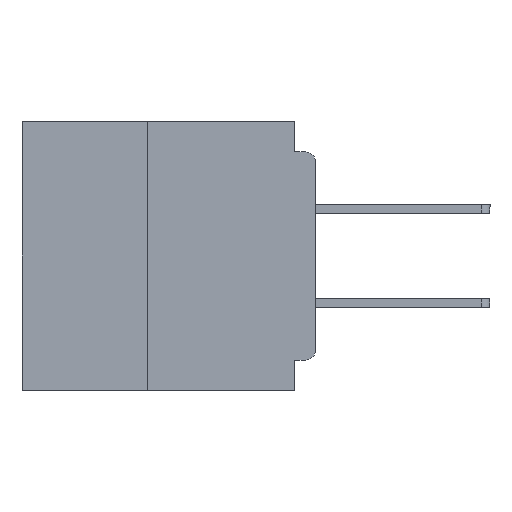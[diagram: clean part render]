
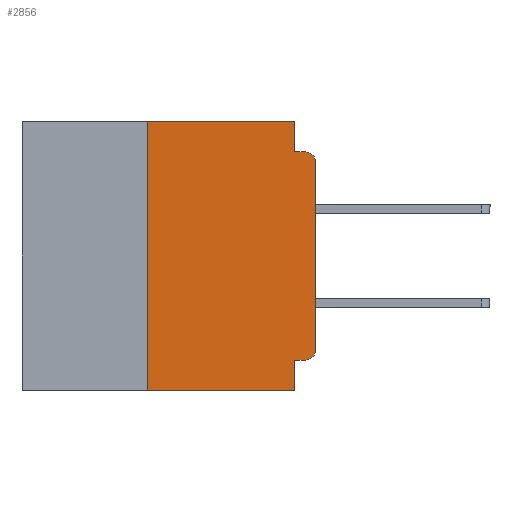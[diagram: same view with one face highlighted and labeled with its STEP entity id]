
A CAD part, left-side view. The second image highlights one B-rep face of the part: STEP entity #2856.
In plain terms, the highlighted planar face has unit normal (-1, 0, 0).
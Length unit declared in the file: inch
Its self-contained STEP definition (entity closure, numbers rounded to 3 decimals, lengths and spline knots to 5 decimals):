
#114 = CARTESIAN_POINT ( 'NONE',  ( 0., 0., 0. ) ) ;
#405 = EDGE_CURVE ( 'NONE', #44280, #7574, #28032, .T. ) ;
#1463 = EDGE_CURVE ( 'NONE', #37430, #23000, #16809, .T. ) ;
#2171 = DIRECTION ( 'NONE',  ( 0., 0., -1. ) ) ;
#2645 = CARTESIAN_POINT ( 'NONE',  ( 0., 0., -0.045 ) ) ;
#2856 = ADVANCED_FACE ( 'NONE', ( #10744 ), #32608, .F. ) ;
#2938 = EDGE_CURVE ( 'NONE', #18710, #21961, #27287, .T. ) ;
#4623 = CIRCLE ( 'NONE', #25023, 0.015 ) ;
#4988 = CARTESIAN_POINT ( 'NONE',  ( 0., 0.437, 0. ) ) ;
#5082 = CARTESIAN_POINT ( 'NONE',  ( 0., 0.015, -0.355 ) ) ;
#5826 = LINE ( 'NONE', #114, #45745 ) ;
#6076 = ORIENTED_EDGE ( 'NONE', *, *, #46661, .T. ) ;
#6151 = LINE ( 'NONE', #39834, #42581 ) ;
#6494 = CARTESIAN_POINT ( 'NONE',  ( 0., 0., -0.355 ) ) ;
#6638 = ORIENTED_EDGE ( 'NONE', *, *, #2938, .F. ) ;
#7228 = VECTOR ( 'NONE', #45148, 39.37008 ) ;
#7574 = VERTEX_POINT ( 'NONE', #24843 ) ;
#7964 = VERTEX_POINT ( 'NONE', #11908 ) ;
#7988 = VECTOR ( 'NONE', #12850, 39.37008 ) ;
#8769 = DIRECTION ( 'NONE',  ( 0., -1., 0. ) ) ;
#10744 = FACE_OUTER_BOUND ( 'NONE', #28054, .T. ) ;
#10746 = ORIENTED_EDGE ( 'NONE', *, *, #1463, .F. ) ;
#10766 = CARTESIAN_POINT ( 'NONE',  ( 0., 0.015, -0.06 ) ) ;
#10974 = LINE ( 'NONE', #35877, #28697 ) ;
#11908 = CARTESIAN_POINT ( 'NONE',  ( 0., 0., -0.34 ) ) ;
#11977 = VERTEX_POINT ( 'NONE', #30404 ) ;
#12850 = DIRECTION ( 'NONE',  ( 0., 0., 1. ) ) ;
#12955 = CARTESIAN_POINT ( 'NONE',  ( 0., 0.031, -0.355 ) ) ;
#13280 = DIRECTION ( 'NONE',  ( 0., -1., 0. ) ) ;
#13637 = ORIENTED_EDGE ( 'NONE', *, *, #16583, .F. ) ;
#13921 = VECTOR ( 'NONE', #36580, 39.37008 ) ;
#14238 = CARTESIAN_POINT ( 'NONE',  ( 0., 0.031, 0. ) ) ;
#14565 = DIRECTION ( 'NONE',  ( 0., 0., -1. ) ) ;
#16583 = EDGE_CURVE ( 'NONE', #21961, #11977, #24001, .T. ) ;
#16809 = LINE ( 'NONE', #6494, #35683 ) ;
#18105 = LINE ( 'NONE', #4988, #46826 ) ;
#18710 = VERTEX_POINT ( 'NONE', #14238 ) ;
#19226 = VERTEX_POINT ( 'NONE', #39712 ) ;
#21714 = DIRECTION ( 'NONE',  ( -1., 0., 0. ) ) ;
#21961 = VERTEX_POINT ( 'NONE', #28727 ) ;
#23000 = VERTEX_POINT ( 'NONE', #12955 ) ;
#24001 = LINE ( 'NONE', #2645, #13921 ) ;
#24843 = CARTESIAN_POINT ( 'NONE',  ( 0., 0.25, 0. ) ) ;
#25023 = AXIS2_PLACEMENT_3D ( 'NONE', #44148, #21714, #47882 ) ;
#25520 = ORIENTED_EDGE ( 'NONE', *, *, #27653, .T. ) ;
#25661 = AXIS2_PLACEMENT_3D ( 'NONE', #10766, #37137, #14565 ) ;
#26467 = DIRECTION ( 'NONE',  ( 0., 0., 1. ) ) ;
#27287 = LINE ( 'NONE', #42027, #7228 ) ;
#27653 = EDGE_CURVE ( 'NONE', #37430, #7964, #4623, .T. ) ;
#28032 = LINE ( 'NONE', #30200, #7988 ) ;
#28054 = EDGE_LOOP ( 'NONE', ( #35463, #41306, #13637, #6638, #30196, #43670, #6076, #29627, #10746, #25520 ) ) ;
#28311 = CIRCLE ( 'NONE', #25661, 0.015 ) ;
#28697 = VECTOR ( 'NONE', #13280, 39.37008 ) ;
#28727 = CARTESIAN_POINT ( 'NONE',  ( 0., 0.031, -0.045 ) ) ;
#29331 = CARTESIAN_POINT ( 'NONE',  ( 0., 0.25, -0.4 ) ) ;
#29627 = ORIENTED_EDGE ( 'NONE', *, *, #41688, .F. ) ;
#30196 = ORIENTED_EDGE ( 'NONE', *, *, #40112, .F. ) ;
#30200 = CARTESIAN_POINT ( 'NONE',  ( 0., 0.25, -0.4 ) ) ;
#30404 = CARTESIAN_POINT ( 'NONE',  ( 0., 0.015, -0.045 ) ) ;
#32608 = PLANE ( 'NONE',  #45919 ) ;
#35463 = ORIENTED_EDGE ( 'NONE', *, *, #39303, .T. ) ;
#35683 = VECTOR ( 'NONE', #41032, 39.37008 ) ;
#35877 = CARTESIAN_POINT ( 'NONE',  ( 0., 0.437, -0.4 ) ) ;
#36580 = DIRECTION ( 'NONE',  ( 0., -1., 0. ) ) ;
#37137 = DIRECTION ( 'NONE',  ( -1., 0., 0. ) ) ;
#37430 = VERTEX_POINT ( 'NONE', #5082 ) ;
#37735 = EDGE_CURVE ( 'NONE', #19226, #11977, #28311, .T. ) ;
#39303 = EDGE_CURVE ( 'NONE', #7964, #19226, #5826, .T. ) ;
#39356 = DIRECTION ( 'NONE',  ( 0., 0., -1. ) ) ;
#39366 = DIRECTION ( 'NONE',  ( 1., 0., 0. ) ) ;
#39410 = CARTESIAN_POINT ( 'NONE',  ( 0., 0.437, 0. ) ) ;
#39712 = CARTESIAN_POINT ( 'NONE',  ( 0., 0., -0.06 ) ) ;
#39834 = CARTESIAN_POINT ( 'NONE',  ( 0., 0.031, -0.4 ) ) ;
#40112 = EDGE_CURVE ( 'NONE', #7574, #18710, #18105, .T. ) ;
#41002 = VERTEX_POINT ( 'NONE', #48391 ) ;
#41032 = DIRECTION ( 'NONE',  ( 0., 1., 0. ) ) ;
#41306 = ORIENTED_EDGE ( 'NONE', *, *, #37735, .T. ) ;
#41688 = EDGE_CURVE ( 'NONE', #23000, #41002, #6151, .T. ) ;
#42027 = CARTESIAN_POINT ( 'NONE',  ( 0., 0.031, 0. ) ) ;
#42581 = VECTOR ( 'NONE', #2171, 39.37008 ) ;
#43670 = ORIENTED_EDGE ( 'NONE', *, *, #405, .F. ) ;
#44148 = CARTESIAN_POINT ( 'NONE',  ( 0., 0.015, -0.34 ) ) ;
#44280 = VERTEX_POINT ( 'NONE', #29331 ) ;
#45148 = DIRECTION ( 'NONE',  ( 0., 0., -1. ) ) ;
#45745 = VECTOR ( 'NONE', #26467, 39.37008 ) ;
#45919 = AXIS2_PLACEMENT_3D ( 'NONE', #39410, #39366, #39356 ) ;
#46661 = EDGE_CURVE ( 'NONE', #44280, #41002, #10974, .T. ) ;
#46826 = VECTOR ( 'NONE', #8769, 39.37008 ) ;
#47882 = DIRECTION ( 'NONE',  ( 0., 0., -1. ) ) ;
#48391 = CARTESIAN_POINT ( 'NONE',  ( 0., 0.031, -0.4 ) ) ;
